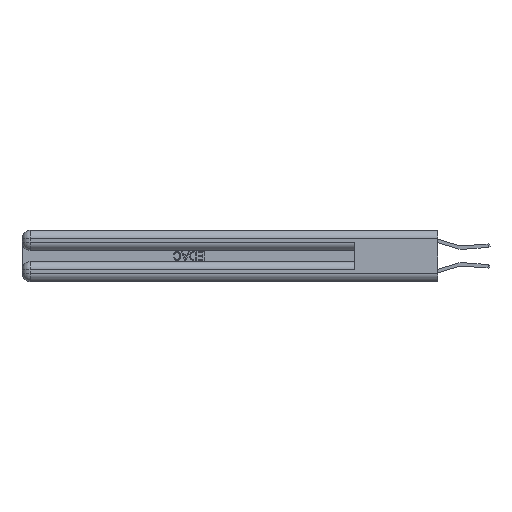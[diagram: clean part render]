
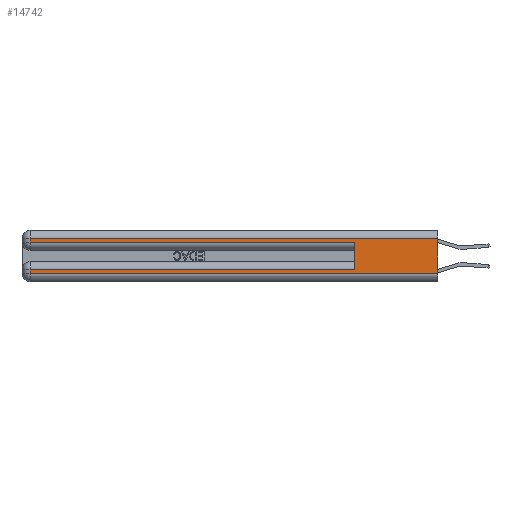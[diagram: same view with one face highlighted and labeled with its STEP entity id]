
A CAD part, left-side view. The second image highlights one B-rep face of the part: STEP entity #14742.
In plain terms, the highlighted planar face has unit normal (-1, 0, 0).
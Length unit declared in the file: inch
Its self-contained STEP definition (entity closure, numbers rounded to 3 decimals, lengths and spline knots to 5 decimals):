
#2069 = ORIENTED_EDGE ( 'NONE', *, *, #6256, .F. ) ;
#2493 = EDGE_CURVE ( 'NONE', #30623, #29063, #6696, .T. ) ;
#2812 = VECTOR ( 'NONE', #21014, 39.37008 ) ;
#2913 = EDGE_CURVE ( 'NONE', #30623, #3943, #22875, .T. ) ;
#3648 = AXIS2_PLACEMENT_3D ( 'NONE', #18663, #9170, #14014 ) ;
#3943 = VERTEX_POINT ( 'NONE', #26632 ) ;
#3974 = VECTOR ( 'NONE', #19897, 39.37008 ) ;
#4066 = ORIENTED_EDGE ( 'NONE', *, *, #7604, .T. ) ;
#4871 = ORIENTED_EDGE ( 'NONE', *, *, #2913, .F. ) ;
#5074 = CARTESIAN_POINT ( 'NONE',  ( 0., 2.94, 0.31 ) ) ;
#5808 = LINE ( 'NONE', #21237, #2812 ) ;
#5922 = CARTESIAN_POINT ( 'NONE',  ( 0., 0., 0.085 ) ) ;
#5983 = CARTESIAN_POINT ( 'NONE',  ( 0., 2.94, 0.085 ) ) ;
#6256 = EDGE_CURVE ( 'NONE', #17370, #24868, #17283, .T. ) ;
#6696 = LINE ( 'NONE', #5922, #20653 ) ;
#7048 = VECTOR ( 'NONE', #10425, 39.37008 ) ;
#7604 = EDGE_CURVE ( 'NONE', #19009, #3943, #24651, .T. ) ;
#7716 = ORIENTED_EDGE ( 'NONE', *, *, #16348, .T. ) ;
#8969 = PLANE ( 'NONE',  #3648 ) ;
#9170 = DIRECTION ( 'NONE',  ( 1., 0., 0. ) ) ;
#9276 = VECTOR ( 'NONE', #19336, 39.37008 ) ;
#9647 = LINE ( 'NONE', #21427, #20581 ) ;
#10425 = DIRECTION ( 'NONE',  ( 0., 0., 1. ) ) ;
#10689 = EDGE_LOOP ( 'NONE', ( #2069, #7716, #24090, #4066, #4871, #19988, #30512, #30319 ) ) ;
#13038 = CARTESIAN_POINT ( 'NONE',  ( 0., 2.94, 0.06 ) ) ;
#14014 = DIRECTION ( 'NONE',  ( 0., 0., -1. ) ) ;
#14742 = ADVANCED_FACE ( 'NONE', ( #17260 ), #8969, .F. ) ;
#15498 = CARTESIAN_POINT ( 'NONE',  ( 0., 0., 0.06 ) ) ;
#15614 = DIRECTION ( 'NONE',  ( 0., 1., 0. ) ) ;
#15764 = CARTESIAN_POINT ( 'NONE',  ( 0., 0.6, 0.085 ) ) ;
#15821 = DIRECTION ( 'NONE',  ( 0., -1., 0. ) ) ;
#15835 = CARTESIAN_POINT ( 'NONE',  ( 0., 0., 0.31 ) ) ;
#16348 = EDGE_CURVE ( 'NONE', #17370, #19200, #5808, .T. ) ;
#16756 = DIRECTION ( 'NONE',  ( 0., 0., -1. ) ) ;
#16777 = DIRECTION ( 'NONE',  ( 0., 0., -1. ) ) ;
#17260 = FACE_OUTER_BOUND ( 'NONE', #10689, .T. ) ;
#17283 = LINE ( 'NONE', #20668, #18030 ) ;
#17345 = CARTESIAN_POINT ( 'NONE',  ( 0., 2.94, 0.37 ) ) ;
#17370 = VERTEX_POINT ( 'NONE', #15835 ) ;
#18030 = VECTOR ( 'NONE', #16756, 39.37008 ) ;
#18663 = CARTESIAN_POINT ( 'NONE',  ( 0., 0., 0.37 ) ) ;
#19009 = VERTEX_POINT ( 'NONE', #26462 ) ;
#19200 = VERTEX_POINT ( 'NONE', #5074 ) ;
#19336 = DIRECTION ( 'NONE',  ( 0., 0., -1. ) ) ;
#19403 = EDGE_CURVE ( 'NONE', #26992, #24868, #21888, .T. ) ;
#19897 = DIRECTION ( 'NONE',  ( 0., -1., 0. ) ) ;
#19988 = ORIENTED_EDGE ( 'NONE', *, *, #2493, .T. ) ;
#20581 = VECTOR ( 'NONE', #16777, 39.37008 ) ;
#20653 = VECTOR ( 'NONE', #15614, 39.37008 ) ;
#20668 = CARTESIAN_POINT ( 'NONE',  ( 0., 0., 0.37 ) ) ;
#21014 = DIRECTION ( 'NONE',  ( 0., 1., 0. ) ) ;
#21237 = CARTESIAN_POINT ( 'NONE',  ( 0., 0., 0.31 ) ) ;
#21427 = CARTESIAN_POINT ( 'NONE',  ( 0., 2.94, 0.37 ) ) ;
#21888 = LINE ( 'NONE', #15498, #27161 ) ;
#22323 = CARTESIAN_POINT ( 'NONE',  ( 0., 0.6, 0.145 ) ) ;
#22875 = LINE ( 'NONE', #22323, #7048 ) ;
#23085 = EDGE_CURVE ( 'NONE', #29063, #26992, #24668, .T. ) ;
#24090 = ORIENTED_EDGE ( 'NONE', *, *, #31139, .T. ) ;
#24494 = CARTESIAN_POINT ( 'NONE',  ( 0., 0., 0.285 ) ) ;
#24651 = LINE ( 'NONE', #24494, #3974 ) ;
#24668 = LINE ( 'NONE', #17345, #9276 ) ;
#24868 = VERTEX_POINT ( 'NONE', #27260 ) ;
#26462 = CARTESIAN_POINT ( 'NONE',  ( 0., 2.94, 0.285 ) ) ;
#26632 = CARTESIAN_POINT ( 'NONE',  ( 0., 0.6, 0.285 ) ) ;
#26992 = VERTEX_POINT ( 'NONE', #13038 ) ;
#27161 = VECTOR ( 'NONE', #15821, 39.37008 ) ;
#27260 = CARTESIAN_POINT ( 'NONE',  ( 0., 0., 0.06 ) ) ;
#29063 = VERTEX_POINT ( 'NONE', #5983 ) ;
#30319 = ORIENTED_EDGE ( 'NONE', *, *, #19403, .T. ) ;
#30512 = ORIENTED_EDGE ( 'NONE', *, *, #23085, .T. ) ;
#30623 = VERTEX_POINT ( 'NONE', #15764 ) ;
#31139 = EDGE_CURVE ( 'NONE', #19200, #19009, #9647, .T. ) ;
